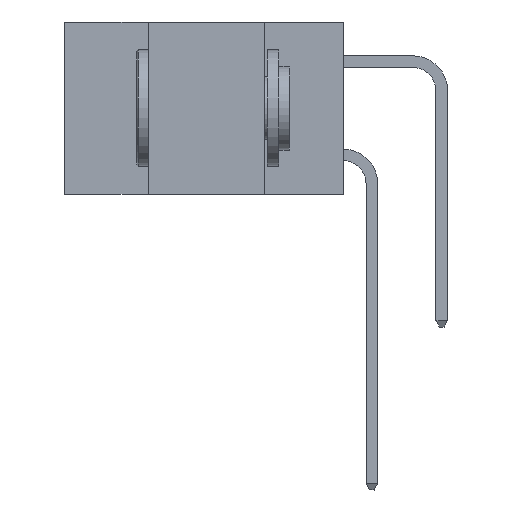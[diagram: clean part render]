
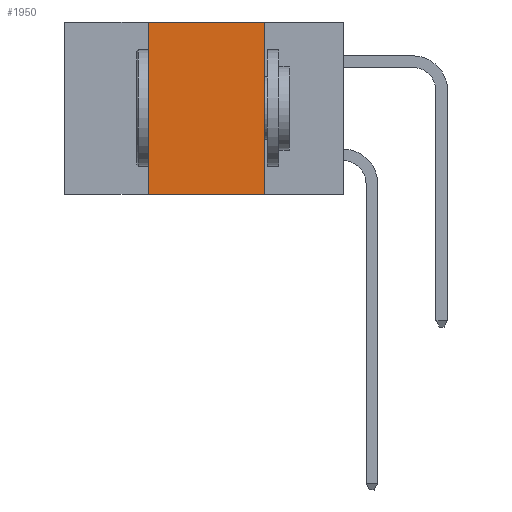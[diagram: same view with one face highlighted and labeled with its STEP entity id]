
A CAD part, left-side view. The second image highlights one B-rep face of the part: STEP entity #1950.
In plain terms, the highlighted planar face has unit normal (-1, 0, 0).
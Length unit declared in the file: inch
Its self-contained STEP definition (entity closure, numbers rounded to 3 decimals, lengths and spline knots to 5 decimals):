
#1435 = FACE_OUTER_BOUND ( 'NONE', #21365, .T. ) ;
#1950 = ADVANCED_FACE ( 'NONE', ( #1435 ), #11988, .F. ) ;
#2135 = EDGE_CURVE ( 'NONE', #14476, #11692, #17896, .T. ) ;
#2569 = CARTESIAN_POINT ( 'NONE',  ( 0., 0.42, -0.37 ) ) ;
#3645 = EDGE_CURVE ( 'NONE', #21508, #15452, #8667, .T. ) ;
#3664 = VECTOR ( 'NONE', #14125, 39.37008 ) ;
#4252 = LINE ( 'NONE', #13572, #3664 ) ;
#4323 = VECTOR ( 'NONE', #17208, 39.37008 ) ;
#4553 = EDGE_CURVE ( 'NONE', #14476, #15452, #4252, .T. ) ;
#6193 = DIRECTION ( 'NONE',  ( 0., 0., 1. ) ) ;
#7684 = CARTESIAN_POINT ( 'NONE',  ( 0., 0.17, 0. ) ) ;
#8267 = ORIENTED_EDGE ( 'NONE', *, *, #23643, .F. ) ;
#8628 = DIRECTION ( 'NONE',  ( 0., -1., 0. ) ) ;
#8629 = CARTESIAN_POINT ( 'NONE',  ( 0., 0.42, 0. ) ) ;
#8667 = LINE ( 'NONE', #7684, #4323 ) ;
#8941 = VECTOR ( 'NONE', #8628, 39.37008 ) ;
#8978 = CARTESIAN_POINT ( 'NONE',  ( 0., 0.17, -0.37 ) ) ;
#10997 = CARTESIAN_POINT ( 'NONE',  ( 0., 0.17, 0. ) ) ;
#11692 = VERTEX_POINT ( 'NONE', #16553 ) ;
#11988 = PLANE ( 'NONE',  #19960 ) ;
#12337 = DIRECTION ( 'NONE',  ( 1., 0., 0. ) ) ;
#12399 = CARTESIAN_POINT ( 'NONE',  ( 0., 0.6, 0. ) ) ;
#13572 = CARTESIAN_POINT ( 'NONE',  ( 0., 0.6, -0.37 ) ) ;
#14125 = DIRECTION ( 'NONE',  ( 0., -1., 0. ) ) ;
#14476 = VERTEX_POINT ( 'NONE', #2569 ) ;
#14601 = LINE ( 'NONE', #16251, #8941 ) ;
#15452 = VERTEX_POINT ( 'NONE', #8978 ) ;
#16251 = CARTESIAN_POINT ( 'NONE',  ( 0., 0.6, 0. ) ) ;
#16553 = CARTESIAN_POINT ( 'NONE',  ( 0., 0.42, 0. ) ) ;
#17208 = DIRECTION ( 'NONE',  ( 0., 0., -1. ) ) ;
#17495 = DIRECTION ( 'NONE',  ( 0., 0., -1. ) ) ;
#17896 = LINE ( 'NONE', #8629, #22191 ) ;
#19960 = AXIS2_PLACEMENT_3D ( 'NONE', #12399, #12337, #17495 ) ;
#20581 = ORIENTED_EDGE ( 'NONE', *, *, #4553, .T. ) ;
#21365 = EDGE_LOOP ( 'NONE', ( #22837, #8267, #23163, #20581 ) ) ;
#21508 = VERTEX_POINT ( 'NONE', #10997 ) ;
#22191 = VECTOR ( 'NONE', #6193, 39.37008 ) ;
#22837 = ORIENTED_EDGE ( 'NONE', *, *, #3645, .F. ) ;
#23163 = ORIENTED_EDGE ( 'NONE', *, *, #2135, .F. ) ;
#23643 = EDGE_CURVE ( 'NONE', #11692, #21508, #14601, .T. ) ;
